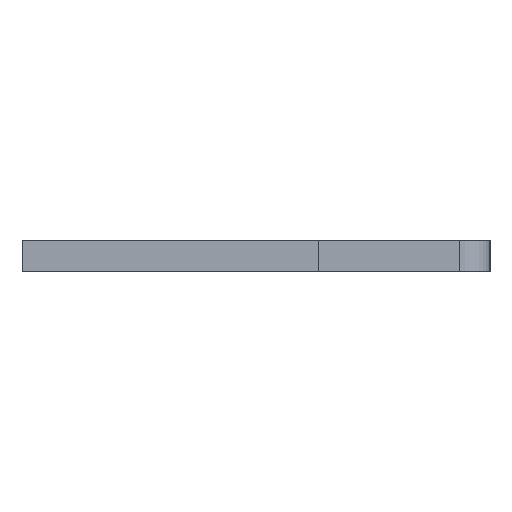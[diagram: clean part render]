
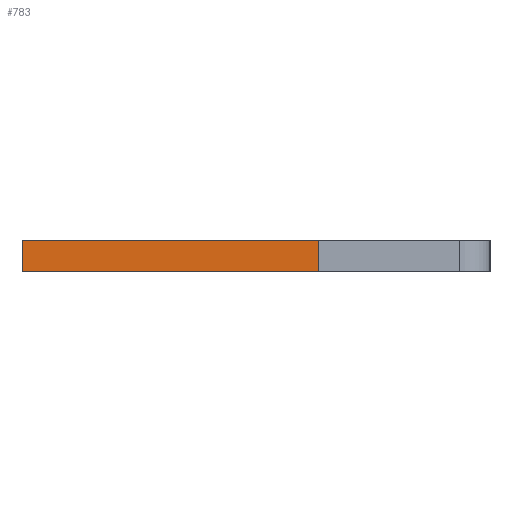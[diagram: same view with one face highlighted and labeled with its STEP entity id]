
A CAD part, left-side view. The second image highlights one B-rep face of the part: STEP entity #783.
In plain terms, the highlighted face is planar.
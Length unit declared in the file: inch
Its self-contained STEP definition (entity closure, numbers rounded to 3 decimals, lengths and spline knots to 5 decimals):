
#78 = EDGE_CURVE ( 'NONE', #1551, #79, #179, .T. ) ;
#79 = VERTEX_POINT ( 'NONE', #379 ) ;
#120 = DIRECTION ( 'NONE',  ( 0., 1., 0. ) ) ;
#162 = AXIS2_PLACEMENT_3D ( 'NONE', #1010, #172, #1526 ) ;
#172 = DIRECTION ( 'NONE',  ( 0., 0., 1. ) ) ;
#179 = LINE ( 'NONE', #965, #1341 ) ;
#187 = DIRECTION ( 'NONE',  ( 0., 1., 0. ) ) ;
#199 = VERTEX_POINT ( 'NONE', #821 ) ;
#241 = VERTEX_POINT ( 'NONE', #433 ) ;
#246 = FACE_OUTER_BOUND ( 'NONE', #1392, .T. ) ;
#378 = CARTESIAN_POINT ( 'NONE',  ( -0.01, -0.04, -0.04 ) ) ;
#379 = CARTESIAN_POINT ( 'NONE',  ( -0.01, 0.15, -0.04 ) ) ;
#381 = EDGE_CURVE ( 'NONE', #199, #79, #757, .T. ) ;
#433 = CARTESIAN_POINT ( 'NONE',  ( 0.01, -0.04, -0.04 ) ) ;
#436 = PLANE ( 'NONE',  #162 ) ;
#445 = LINE ( 'NONE', #903, #1677 ) ;
#491 = ORIENTED_EDGE ( 'NONE', *, *, #78, .T. ) ;
#709 = DIRECTION ( 'NONE',  ( -1., 0., 0. ) ) ;
#757 = LINE ( 'NONE', #1251, #1619 ) ;
#783 = ADVANCED_FACE ( 'NONE', ( #246 ), #436, .F. ) ;
#821 = CARTESIAN_POINT ( 'NONE',  ( 0.01, 0.15, -0.04 ) ) ;
#903 = CARTESIAN_POINT ( 'NONE',  ( 0.01, 0.15, -0.04 ) ) ;
#965 = CARTESIAN_POINT ( 'NONE',  ( -0.01, 0.15, -0.04 ) ) ;
#1010 = CARTESIAN_POINT ( 'NONE',  ( 0.01, 0.15, -0.04 ) ) ;
#1064 = ORIENTED_EDGE ( 'NONE', *, *, #381, .F. ) ;
#1111 = VECTOR ( 'NONE', #1593, 39.37008 ) ;
#1165 = EDGE_CURVE ( 'NONE', #241, #199, #445, .T. ) ;
#1194 = CARTESIAN_POINT ( 'NONE',  ( 0.01, -0.04, -0.04 ) ) ;
#1251 = CARTESIAN_POINT ( 'NONE',  ( 0.01, 0.15, -0.04 ) ) ;
#1339 = ORIENTED_EDGE ( 'NONE', *, *, #1373, .T. ) ;
#1341 = VECTOR ( 'NONE', #120, 39.37008 ) ;
#1373 = EDGE_CURVE ( 'NONE', #241, #1551, #1472, .T. ) ;
#1392 = EDGE_LOOP ( 'NONE', ( #491, #1064, #1577, #1339 ) ) ;
#1472 = LINE ( 'NONE', #1194, #1111 ) ;
#1526 = DIRECTION ( 'NONE',  ( 1., 0., 0. ) ) ;
#1551 = VERTEX_POINT ( 'NONE', #378 ) ;
#1577 = ORIENTED_EDGE ( 'NONE', *, *, #1165, .F. ) ;
#1593 = DIRECTION ( 'NONE',  ( -1., 0., 0. ) ) ;
#1619 = VECTOR ( 'NONE', #709, 39.37008 ) ;
#1677 = VECTOR ( 'NONE', #187, 39.37008 ) ;
